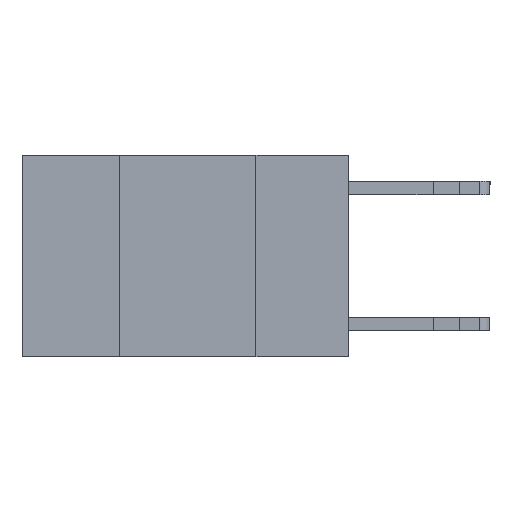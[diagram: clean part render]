
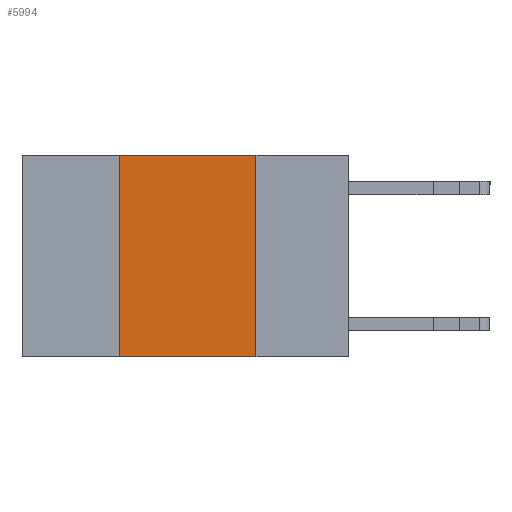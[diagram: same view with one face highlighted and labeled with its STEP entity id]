
A CAD part, left-side view. The second image highlights one B-rep face of the part: STEP entity #5994.
In plain terms, the highlighted planar face has unit normal (-1, 0, 0).
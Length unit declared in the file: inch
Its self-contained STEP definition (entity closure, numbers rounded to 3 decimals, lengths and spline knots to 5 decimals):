
#687 = LINE ( 'NONE', #20324, #8509 ) ;
#3510 = CARTESIAN_POINT ( 'NONE',  ( 0., 0.42, -0.37 ) ) ;
#4399 = ORIENTED_EDGE ( 'NONE', *, *, #11015, .T. ) ;
#4739 = LINE ( 'NONE', #13852, #18277 ) ;
#5081 = DIRECTION ( 'NONE',  ( 0., 0., -1. ) ) ;
#5994 = ADVANCED_FACE ( 'NONE', ( #7713 ), #10045, .F. ) ;
#7503 = ORIENTED_EDGE ( 'NONE', *, *, #13182, .F. ) ;
#7713 = FACE_OUTER_BOUND ( 'NONE', #18481, .T. ) ;
#7840 = VERTEX_POINT ( 'NONE', #3510 ) ;
#8509 = VECTOR ( 'NONE', #5081, 39.37008 ) ;
#10045 = PLANE ( 'NONE',  #12218 ) ;
#10565 = CARTESIAN_POINT ( 'NONE',  ( 0., 0.42, 0. ) ) ;
#10706 = VERTEX_POINT ( 'NONE', #10565 ) ;
#11015 = EDGE_CURVE ( 'NONE', #7840, #20631, #4739, .T. ) ;
#11494 = CARTESIAN_POINT ( 'NONE',  ( 0., 0.17, -0.37 ) ) ;
#11768 = CARTESIAN_POINT ( 'NONE',  ( 0., 0.17, 0. ) ) ;
#12218 = AXIS2_PLACEMENT_3D ( 'NONE', #14518, #23812, #25869 ) ;
#12383 = ORIENTED_EDGE ( 'NONE', *, *, #22503, .F. ) ;
#13182 = EDGE_CURVE ( 'NONE', #16573, #20631, #687, .T. ) ;
#13379 = LINE ( 'NONE', #22520, #27264 ) ;
#13852 = CARTESIAN_POINT ( 'NONE',  ( 0., 0.6, -0.37 ) ) ;
#14518 = CARTESIAN_POINT ( 'NONE',  ( 0., 0.6, 0. ) ) ;
#14963 = CARTESIAN_POINT ( 'NONE',  ( 0., 0.42, 0. ) ) ;
#16417 = VECTOR ( 'NONE', #19636, 39.37008 ) ;
#16573 = VERTEX_POINT ( 'NONE', #11768 ) ;
#18229 = ORIENTED_EDGE ( 'NONE', *, *, #27526, .F. ) ;
#18277 = VECTOR ( 'NONE', #18515, 39.37008 ) ;
#18481 = EDGE_LOOP ( 'NONE', ( #7503, #12383, #18229, #4399 ) ) ;
#18515 = DIRECTION ( 'NONE',  ( 0., -1., 0. ) ) ;
#19636 = DIRECTION ( 'NONE',  ( 0., 0., 1. ) ) ;
#20324 = CARTESIAN_POINT ( 'NONE',  ( 0., 0.17, 0. ) ) ;
#20631 = VERTEX_POINT ( 'NONE', #11494 ) ;
#22230 = DIRECTION ( 'NONE',  ( 0., -1., 0. ) ) ;
#22503 = EDGE_CURVE ( 'NONE', #10706, #16573, #13379, .T. ) ;
#22520 = CARTESIAN_POINT ( 'NONE',  ( 0., 0.6, 0. ) ) ;
#23812 = DIRECTION ( 'NONE',  ( 1., 0., 0. ) ) ;
#25869 = DIRECTION ( 'NONE',  ( 0., 0., -1. ) ) ;
#26028 = LINE ( 'NONE', #14963, #16417 ) ;
#27264 = VECTOR ( 'NONE', #22230, 39.37008 ) ;
#27526 = EDGE_CURVE ( 'NONE', #7840, #10706, #26028, .T. ) ;
